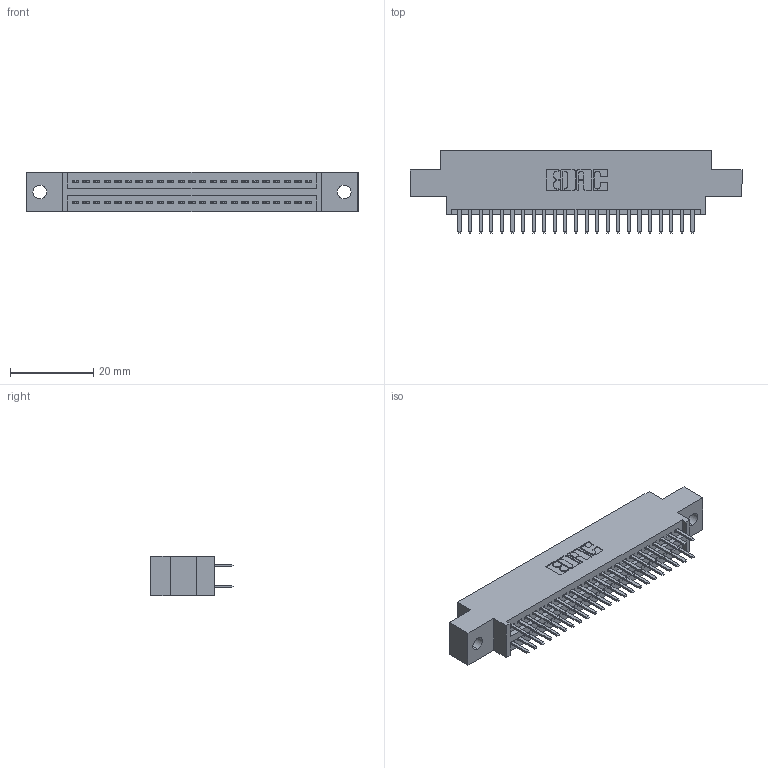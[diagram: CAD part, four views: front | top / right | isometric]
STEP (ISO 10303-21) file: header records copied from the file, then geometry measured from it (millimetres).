
FILE_DESCRIPTION (( 'STEP AP203' ), '1' );
FILE_NAME ('345-046-520-802.STEP', '2019-10-29T01:20:00', ( '' ), ( '' ), 'SwSTEP 2.0', 'SolidWorks 2016', '' );
FILE_SCHEMA (( 'CONFIG_CONTROL_DESIGN' ));
Length unit declared in the file: inch
Products named in the file (3): 345 Part_0.170 Offset - 0.128 Dia; 345-292-001_345-293-120; 345-046-520-802
Assembly tree (47 placements, depth 2):
  345-046-520-802
    345 Part_0.170 Offset - 0.128 Dia
    345-292-001_345-293-120  x46
Bounding box: 79.63 x 19.68 x 9.4 mm (x, y, z)
Volume: 7388.6 mm3; surface area: 10381.3 mm2
Topology: 47 solids, 47 shells, 2614 faces, 7575 edges, 4926 vertices
Faces by surface type: plane 1694, cylinder 920
Entity records: 20853 total; most frequent: CARTESIAN_POINT 3528, ORIENTED_EDGE 3450, DIRECTION 3121, EDGE_CURVE 1725, LINE 1497, VECTOR 1497, VERTEX_POINT 1146, AXIS2_PLACEMENT_3D 812
